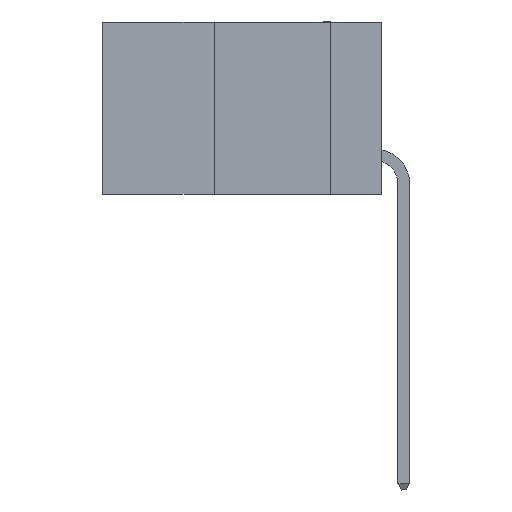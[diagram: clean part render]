
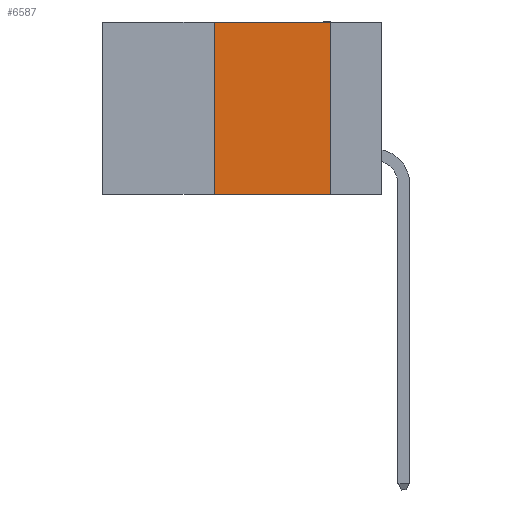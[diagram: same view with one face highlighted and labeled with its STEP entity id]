
A CAD part, left-side view. The second image highlights one B-rep face of the part: STEP entity #6587.
In plain terms, the highlighted planar face has unit normal (-1, 0, 0).
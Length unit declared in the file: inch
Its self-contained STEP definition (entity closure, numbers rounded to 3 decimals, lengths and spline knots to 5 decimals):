
#2450 = EDGE_LOOP ( 'NONE', ( #10506, #13803, #10399, #10482 ) ) ;
#6362 = PLANE ( 'NONE',  #6581 ) ;
#6581 = AXIS2_PLACEMENT_3D ( 'NONE', #24613, #27649, #9374 ) ;
#6587 = ADVANCED_FACE ( 'NONE', ( #34502 ), #6362, .F. ) ;
#9374 = DIRECTION ( 'NONE',  ( 0., 0., -1. ) ) ;
#9454 = CARTESIAN_POINT ( 'NONE',  ( 0., 0.11, -0.37 ) ) ;
#10399 = ORIENTED_EDGE ( 'NONE', *, *, #36641, .F. ) ;
#10415 = LINE ( 'NONE', #22477, #17559 ) ;
#10482 = ORIENTED_EDGE ( 'NONE', *, *, #38645, .T. ) ;
#10506 = ORIENTED_EDGE ( 'NONE', *, *, #26741, .F. ) ;
#11644 = CARTESIAN_POINT ( 'NONE',  ( 0., 0.36, 0. ) ) ;
#12114 = VECTOR ( 'NONE', #23812, 39.37008 ) ;
#13317 = DIRECTION ( 'NONE',  ( 0., 0., 1. ) ) ;
#13803 = ORIENTED_EDGE ( 'NONE', *, *, #22436, .F. ) ;
#15387 = VERTEX_POINT ( 'NONE', #9454 ) ;
#16178 = VECTOR ( 'NONE', #34612, 39.37008 ) ;
#17559 = VECTOR ( 'NONE', #13317, 39.37008 ) ;
#18124 = VECTOR ( 'NONE', #19712, 39.37008 ) ;
#18251 = CARTESIAN_POINT ( 'NONE',  ( 0., 0.36, -0.37 ) ) ;
#18258 = VERTEX_POINT ( 'NONE', #18251 ) ;
#18409 = VERTEX_POINT ( 'NONE', #19181 ) ;
#19181 = CARTESIAN_POINT ( 'NONE',  ( 0., 0.11, 0. ) ) ;
#19712 = DIRECTION ( 'NONE',  ( 0., -1., 0. ) ) ;
#20529 = VERTEX_POINT ( 'NONE', #11644 ) ;
#20757 = CARTESIAN_POINT ( 'NONE',  ( 0., 0.6, -0.37 ) ) ;
#21249 = LINE ( 'NONE', #20757, #12114 ) ;
#22436 = EDGE_CURVE ( 'NONE', #20529, #18409, #27181, .T. ) ;
#22477 = CARTESIAN_POINT ( 'NONE',  ( 0., 0.36, 0. ) ) ;
#23812 = DIRECTION ( 'NONE',  ( 0., -1., 0. ) ) ;
#24310 = LINE ( 'NONE', #37474, #16178 ) ;
#24613 = CARTESIAN_POINT ( 'NONE',  ( 0., 0.6, 0. ) ) ;
#26741 = EDGE_CURVE ( 'NONE', #18409, #15387, #24310, .T. ) ;
#27181 = LINE ( 'NONE', #31808, #18124 ) ;
#27649 = DIRECTION ( 'NONE',  ( 1., 0., 0. ) ) ;
#31808 = CARTESIAN_POINT ( 'NONE',  ( 0., 0.6, 0. ) ) ;
#34502 = FACE_OUTER_BOUND ( 'NONE', #2450, .T. ) ;
#34612 = DIRECTION ( 'NONE',  ( 0., 0., -1. ) ) ;
#36641 = EDGE_CURVE ( 'NONE', #18258, #20529, #10415, .T. ) ;
#37474 = CARTESIAN_POINT ( 'NONE',  ( 0., 0.11, 0. ) ) ;
#38645 = EDGE_CURVE ( 'NONE', #18258, #15387, #21249, .T. ) ;
